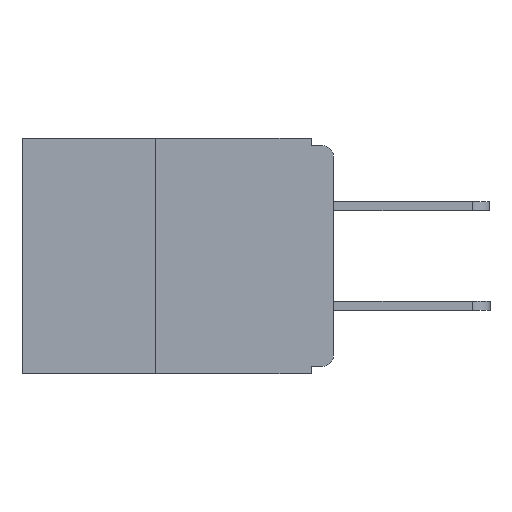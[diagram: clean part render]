
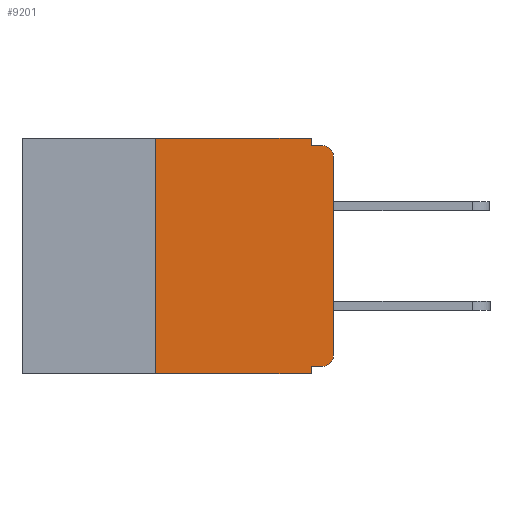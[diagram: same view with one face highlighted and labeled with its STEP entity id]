
A CAD part, left-side view. The second image highlights one B-rep face of the part: STEP entity #9201.
In plain terms, the highlighted planar face has unit normal (-1, 0, 0).
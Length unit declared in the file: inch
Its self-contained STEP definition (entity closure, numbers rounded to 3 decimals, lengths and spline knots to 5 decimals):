
#231 = ORIENTED_EDGE ( 'NONE', *, *, #1196, .T. ) ;
#1085 = EDGE_CURVE ( 'NONE', #25097, #33237, #31575, .T. ) ;
#1196 = EDGE_CURVE ( 'NONE', #23374, #14513, #7489, .T. ) ;
#1894 = DIRECTION ( 'NONE',  ( 0., 0., 1. ) ) ;
#2174 = ORIENTED_EDGE ( 'NONE', *, *, #5728, .F. ) ;
#2397 = CARTESIAN_POINT ( 'NONE',  ( 0., 0.25, -0.33 ) ) ;
#3275 = EDGE_CURVE ( 'NONE', #23374, #20576, #26292, .T. ) ;
#3462 = CARTESIAN_POINT ( 'NONE',  ( 0., 0.031, -0.33 ) ) ;
#4281 = VECTOR ( 'NONE', #32791, 39.37008 ) ;
#4444 = LINE ( 'NONE', #11099, #31472 ) ;
#4840 = EDGE_LOOP ( 'NONE', ( #19803, #23928, #9360, #11007, #2174, #28245, #29842, #20571, #6172, #231 ) ) ;
#4954 = CARTESIAN_POINT ( 'NONE',  ( 0., 0.015, -0.01 ) ) ;
#5318 = EDGE_CURVE ( 'NONE', #7117, #13368, #9923, .T. ) ;
#5728 = EDGE_CURVE ( 'NONE', #13368, #30676, #4444, .T. ) ;
#5900 = CARTESIAN_POINT ( 'NONE',  ( 0., 0.015, -0.305 ) ) ;
#6172 = ORIENTED_EDGE ( 'NONE', *, *, #3275, .F. ) ;
#6659 = CARTESIAN_POINT ( 'NONE',  ( 0., 0.031, -0.33 ) ) ;
#6713 = DIRECTION ( 'NONE',  ( -1., 0., 0. ) ) ;
#6898 = CARTESIAN_POINT ( 'NONE',  ( 0., 0., -0.025 ) ) ;
#7093 = CARTESIAN_POINT ( 'NONE',  ( 0., 0.015, -0.025 ) ) ;
#7117 = VERTEX_POINT ( 'NONE', #18897 ) ;
#7489 = CIRCLE ( 'NONE', #14543, 0.015 ) ;
#8378 = FACE_OUTER_BOUND ( 'NONE', #4840, .T. ) ;
#9201 = ADVANCED_FACE ( 'NONE', ( #8378 ), #28764, .F. ) ;
#9296 = LINE ( 'NONE', #3462, #15472 ) ;
#9360 = ORIENTED_EDGE ( 'NONE', *, *, #17722, .F. ) ;
#9906 = VECTOR ( 'NONE', #18398, 39.37008 ) ;
#9923 = LINE ( 'NONE', #2397, #16096 ) ;
#10005 = DIRECTION ( 'NONE',  ( 0., -1., 0. ) ) ;
#11007 = ORIENTED_EDGE ( 'NONE', *, *, #22982, .F. ) ;
#11099 = CARTESIAN_POINT ( 'NONE',  ( 0., 0.437, 0. ) ) ;
#11664 = VERTEX_POINT ( 'NONE', #6659 ) ;
#13368 = VERTEX_POINT ( 'NONE', #21585 ) ;
#14513 = VERTEX_POINT ( 'NONE', #16099 ) ;
#14543 = AXIS2_PLACEMENT_3D ( 'NONE', #5900, #6713, #23709 ) ;
#15472 = VECTOR ( 'NONE', #29678, 39.37008 ) ;
#16045 = CARTESIAN_POINT ( 'NONE',  ( 0., 0., -0.01 ) ) ;
#16069 = EDGE_CURVE ( 'NONE', #20576, #11664, #9296, .T. ) ;
#16096 = VECTOR ( 'NONE', #1894, 39.37008 ) ;
#16099 = CARTESIAN_POINT ( 'NONE',  ( 0., 0., -0.305 ) ) ;
#16164 = DIRECTION ( 'NONE',  ( -1., 0., 0. ) ) ;
#16217 = DIRECTION ( 'NONE',  ( 0., 0., -1. ) ) ;
#17239 = CARTESIAN_POINT ( 'NONE',  ( 0., 0.031, -0.01 ) ) ;
#17722 = EDGE_CURVE ( 'NONE', #28449, #33237, #33144, .T. ) ;
#18398 = DIRECTION ( 'NONE',  ( 0., 0., 1. ) ) ;
#18897 = CARTESIAN_POINT ( 'NONE',  ( 0., 0.25, -0.33 ) ) ;
#19803 = ORIENTED_EDGE ( 'NONE', *, *, #22608, .T. ) ;
#20571 = ORIENTED_EDGE ( 'NONE', *, *, #16069, .F. ) ;
#20576 = VERTEX_POINT ( 'NONE', #22112 ) ;
#21047 = CARTESIAN_POINT ( 'NONE',  ( 0., 0., 0. ) ) ;
#21337 = EDGE_CURVE ( 'NONE', #7117, #11664, #32103, .T. ) ;
#21585 = CARTESIAN_POINT ( 'NONE',  ( 0., 0.25, 0. ) ) ;
#22112 = CARTESIAN_POINT ( 'NONE',  ( 0., 0.031, -0.32 ) ) ;
#22608 = EDGE_CURVE ( 'NONE', #14513, #25097, #30716, .T. ) ;
#22982 = EDGE_CURVE ( 'NONE', #30676, #28449, #33805, .T. ) ;
#23374 = VERTEX_POINT ( 'NONE', #29326 ) ;
#23709 = DIRECTION ( 'NONE',  ( 0., 0., -1. ) ) ;
#23928 = ORIENTED_EDGE ( 'NONE', *, *, #1085, .T. ) ;
#25097 = VERTEX_POINT ( 'NONE', #6898 ) ;
#25136 = CARTESIAN_POINT ( 'NONE',  ( 0., 0.031, 0. ) ) ;
#25332 = CARTESIAN_POINT ( 'NONE',  ( 0., 0.031, 0. ) ) ;
#26292 = LINE ( 'NONE', #33230, #33775 ) ;
#26432 = VECTOR ( 'NONE', #31567, 39.37008 ) ;
#27607 = DIRECTION ( 'NONE',  ( 0., 0., -1. ) ) ;
#28131 = DIRECTION ( 'NONE',  ( 0., 1., 0. ) ) ;
#28245 = ORIENTED_EDGE ( 'NONE', *, *, #5318, .F. ) ;
#28449 = VERTEX_POINT ( 'NONE', #17239 ) ;
#28659 = DIRECTION ( 'NONE',  ( 0., 0., -1. ) ) ;
#28727 = DIRECTION ( 'NONE',  ( 1., 0., 0. ) ) ;
#28764 = PLANE ( 'NONE',  #30645 ) ;
#29050 = CARTESIAN_POINT ( 'NONE',  ( 0., 0.437, 0. ) ) ;
#29326 = CARTESIAN_POINT ( 'NONE',  ( 0., 0.015, -0.32 ) ) ;
#29678 = DIRECTION ( 'NONE',  ( 0., 0., -1. ) ) ;
#29842 = ORIENTED_EDGE ( 'NONE', *, *, #21337, .T. ) ;
#30385 = CARTESIAN_POINT ( 'NONE',  ( 0., 0.437, -0.33 ) ) ;
#30645 = AXIS2_PLACEMENT_3D ( 'NONE', #29050, #28727, #28659 ) ;
#30676 = VERTEX_POINT ( 'NONE', #25332 ) ;
#30716 = LINE ( 'NONE', #21047, #9906 ) ;
#31472 = VECTOR ( 'NONE', #10005, 39.37008 ) ;
#31567 = DIRECTION ( 'NONE',  ( 0., -1., 0. ) ) ;
#31575 = CIRCLE ( 'NONE', #32556, 0.015 ) ;
#32103 = LINE ( 'NONE', #30385, #4281 ) ;
#32556 = AXIS2_PLACEMENT_3D ( 'NONE', #7093, #16164, #16217 ) ;
#32791 = DIRECTION ( 'NONE',  ( 0., -1., 0. ) ) ;
#33026 = VECTOR ( 'NONE', #27607, 39.37008 ) ;
#33144 = LINE ( 'NONE', #16045, #26432 ) ;
#33230 = CARTESIAN_POINT ( 'NONE',  ( 0., 0., -0.32 ) ) ;
#33237 = VERTEX_POINT ( 'NONE', #4954 ) ;
#33775 = VECTOR ( 'NONE', #28131, 39.37008 ) ;
#33805 = LINE ( 'NONE', #25136, #33026 ) ;
